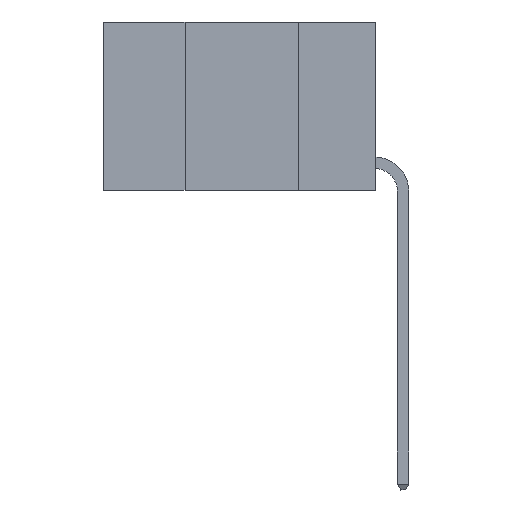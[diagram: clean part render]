
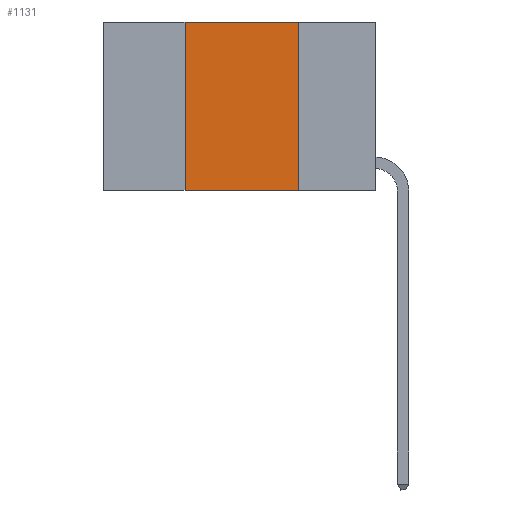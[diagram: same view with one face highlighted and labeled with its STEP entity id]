
A CAD part, left-side view. The second image highlights one B-rep face of the part: STEP entity #1131.
In plain terms, the highlighted planar face has unit normal (-1, 0, 0).
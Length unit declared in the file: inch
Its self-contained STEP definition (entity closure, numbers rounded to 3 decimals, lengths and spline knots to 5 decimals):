
#1131 = ADVANCED_FACE ( 'NONE', ( #21160 ), #1941, .F. ) ;
#1445 = ORIENTED_EDGE ( 'NONE', *, *, #1760, .F. ) ;
#1760 = EDGE_CURVE ( 'NONE', #22728, #13983, #3656, .T. ) ;
#1941 = PLANE ( 'NONE',  #22940 ) ;
#3130 = ORIENTED_EDGE ( 'NONE', *, *, #8143, .F. ) ;
#3656 = LINE ( 'NONE', #16400, #26018 ) ;
#3657 = ORIENTED_EDGE ( 'NONE', *, *, #26587, .T. ) ;
#3793 = DIRECTION ( 'NONE',  ( 0., 0., 1. ) ) ;
#3957 = VECTOR ( 'NONE', #13408, 39.37008 ) ;
#4030 = DIRECTION ( 'NONE',  ( 1., 0., 0. ) ) ;
#4881 = CARTESIAN_POINT ( 'NONE',  ( 0., 0.17, 0. ) ) ;
#5535 = VECTOR ( 'NONE', #26137, 39.37008 ) ;
#6901 = EDGE_LOOP ( 'NONE', ( #3130, #14117, #1445, #3657 ) ) ;
#6993 = VECTOR ( 'NONE', #24886, 39.37008 ) ;
#7983 = CARTESIAN_POINT ( 'NONE',  ( 0., 0.17, -0.37 ) ) ;
#8143 = EDGE_CURVE ( 'NONE', #17134, #9657, #25470, .T. ) ;
#8944 = CARTESIAN_POINT ( 'NONE',  ( 0., 0.42, -0.37 ) ) ;
#9657 = VERTEX_POINT ( 'NONE', #7983 ) ;
#10032 = CARTESIAN_POINT ( 'NONE',  ( 0., 0.17, 0. ) ) ;
#12118 = CARTESIAN_POINT ( 'NONE',  ( 0., 0.42, 0. ) ) ;
#13408 = DIRECTION ( 'NONE',  ( 0., 0., -1. ) ) ;
#13983 = VERTEX_POINT ( 'NONE', #12118 ) ;
#14117 = ORIENTED_EDGE ( 'NONE', *, *, #14988, .F. ) ;
#14602 = LINE ( 'NONE', #18579, #6993 ) ;
#14988 = EDGE_CURVE ( 'NONE', #13983, #17134, #14602, .T. ) ;
#16400 = CARTESIAN_POINT ( 'NONE',  ( 0., 0.42, 0. ) ) ;
#17134 = VERTEX_POINT ( 'NONE', #10032 ) ;
#18579 = CARTESIAN_POINT ( 'NONE',  ( 0., 0.6, 0. ) ) ;
#18830 = DIRECTION ( 'NONE',  ( 0., 0., -1. ) ) ;
#21160 = FACE_OUTER_BOUND ( 'NONE', #6901, .T. ) ;
#22146 = CARTESIAN_POINT ( 'NONE',  ( 0., 0.6, -0.37 ) ) ;
#22278 = LINE ( 'NONE', #22146, #5535 ) ;
#22728 = VERTEX_POINT ( 'NONE', #8944 ) ;
#22801 = CARTESIAN_POINT ( 'NONE',  ( 0., 0.6, 0. ) ) ;
#22940 = AXIS2_PLACEMENT_3D ( 'NONE', #22801, #4030, #18830 ) ;
#24886 = DIRECTION ( 'NONE',  ( 0., -1., 0. ) ) ;
#25470 = LINE ( 'NONE', #4881, #3957 ) ;
#26018 = VECTOR ( 'NONE', #3793, 39.37008 ) ;
#26137 = DIRECTION ( 'NONE',  ( 0., -1., 0. ) ) ;
#26587 = EDGE_CURVE ( 'NONE', #22728, #9657, #22278, .T. ) ;
